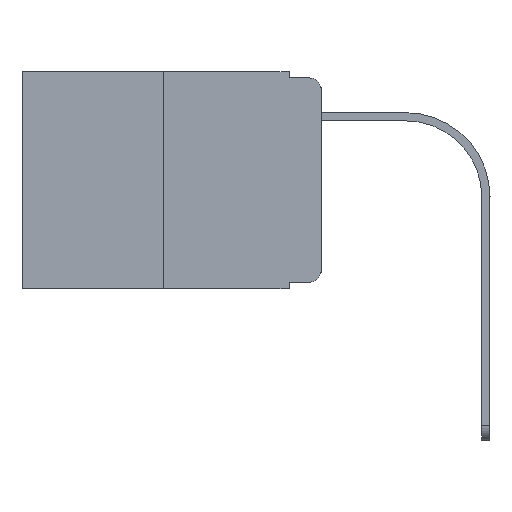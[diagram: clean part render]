
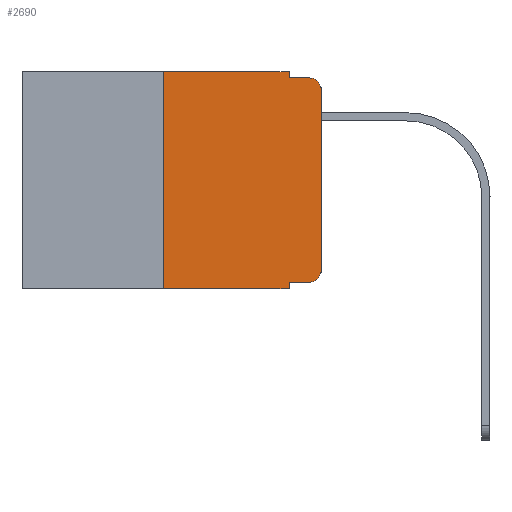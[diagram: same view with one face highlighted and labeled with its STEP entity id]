
A CAD part, left-side view. The second image highlights one B-rep face of the part: STEP entity #2690.
In plain terms, the highlighted planar face has unit normal (-1, 0, 0).
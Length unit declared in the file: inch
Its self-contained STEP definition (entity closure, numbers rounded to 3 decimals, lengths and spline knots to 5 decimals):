
#59 = CARTESIAN_POINT ( 'NONE',  ( 0., 0.051, 0. ) ) ;
#153 = DIRECTION ( 'NONE',  ( -1., 0., 0. ) ) ;
#318 = ORIENTED_EDGE ( 'NONE', *, *, #4493, .F. ) ;
#426 = CARTESIAN_POINT ( 'NONE',  ( 0., 0.473, 0. ) ) ;
#487 = DIRECTION ( 'NONE',  ( 1., 0., 0. ) ) ;
#497 = CIRCLE ( 'NONE', #7524, 0.02 ) ;
#690 = CARTESIAN_POINT ( 'NONE',  ( 0., 0.051, -0.01 ) ) ;
#861 = EDGE_CURVE ( 'NONE', #11144, #884, #11295, .T. ) ;
#884 = VERTEX_POINT ( 'NONE', #4668 ) ;
#1191 = EDGE_CURVE ( 'NONE', #9181, #11509, #8851, .T. ) ;
#1314 = ORIENTED_EDGE ( 'NONE', *, *, #3834, .F. ) ;
#1510 = VECTOR ( 'NONE', #5230, 39.37008 ) ;
#1540 = FACE_OUTER_BOUND ( 'NONE', #5552, .T. ) ;
#1610 = LINE ( 'NONE', #8327, #11600 ) ;
#1935 = ORIENTED_EDGE ( 'NONE', *, *, #7911, .T. ) ;
#2115 = DIRECTION ( 'NONE',  ( 0., 0., -1. ) ) ;
#2291 = LINE ( 'NONE', #8068, #1510 ) ;
#2505 = EDGE_CURVE ( 'NONE', #9447, #11509, #4619, .T. ) ;
#2646 = EDGE_CURVE ( 'NONE', #11144, #7673, #6015, .T. ) ;
#2681 = ORIENTED_EDGE ( 'NONE', *, *, #2850, .T. ) ;
#2690 = ADVANCED_FACE ( 'NONE', ( #1540 ), #9013, .F. ) ;
#2784 = CARTESIAN_POINT ( 'NONE',  ( 0., 0.25, 0. ) ) ;
#2837 = DIRECTION ( 'NONE',  ( 0., 0., -1. ) ) ;
#2850 = EDGE_CURVE ( 'NONE', #11468, #9181, #1610, .T. ) ;
#2859 = CARTESIAN_POINT ( 'NONE',  ( 0., 0., -0.313 ) ) ;
#2957 = CARTESIAN_POINT ( 'NONE',  ( 0., 0.051, 0. ) ) ;
#3092 = CARTESIAN_POINT ( 'NONE',  ( 0., 0.051, 0. ) ) ;
#3671 = ORIENTED_EDGE ( 'NONE', *, *, #1191, .T. ) ;
#3724 = CARTESIAN_POINT ( 'NONE',  ( 0., 0.25, -0.343 ) ) ;
#3834 = EDGE_CURVE ( 'NONE', #8949, #5104, #2291, .T. ) ;
#3927 = DIRECTION ( 'NONE',  ( 0., -1., 0. ) ) ;
#3936 = DIRECTION ( 'NONE',  ( 0., -1., 0. ) ) ;
#4010 = ORIENTED_EDGE ( 'NONE', *, *, #5837, .F. ) ;
#4493 = EDGE_CURVE ( 'NONE', #5104, #10825, #10637, .T. ) ;
#4619 = LINE ( 'NONE', #690, #6845 ) ;
#4668 = CARTESIAN_POINT ( 'NONE',  ( 0., 0.02, -0.333 ) ) ;
#4962 = VECTOR ( 'NONE', #2837, 39.37008 ) ;
#5104 = VERTEX_POINT ( 'NONE', #2784 ) ;
#5146 = DIRECTION ( 'NONE',  ( 0., 0., -1. ) ) ;
#5230 = DIRECTION ( 'NONE',  ( 0., 0., 1. ) ) ;
#5240 = DIRECTION ( 'NONE',  ( 0., 0., -1. ) ) ;
#5477 = ORIENTED_EDGE ( 'NONE', *, *, #6198, .T. ) ;
#5552 = EDGE_LOOP ( 'NONE', ( #2681, #3671, #10069, #4010, #318, #1314, #5477, #10979, #10586, #1935 ) ) ;
#5634 = DIRECTION ( 'NONE',  ( 0., -1., 0. ) ) ;
#5811 = CARTESIAN_POINT ( 'NONE',  ( 0., 0.02, -0.01 ) ) ;
#5837 = EDGE_CURVE ( 'NONE', #10825, #9447, #11525, .T. ) ;
#5990 = VECTOR ( 'NONE', #3927, 39.37008 ) ;
#6015 = LINE ( 'NONE', #59, #7045 ) ;
#6198 = EDGE_CURVE ( 'NONE', #8949, #7673, #10458, .T. ) ;
#6517 = DIRECTION ( 'NONE',  ( 0., -1., 0. ) ) ;
#6740 = VECTOR ( 'NONE', #3936, 39.37008 ) ;
#6845 = VECTOR ( 'NONE', #5634, 39.37008 ) ;
#7017 = CARTESIAN_POINT ( 'NONE',  ( 0., 0.051, -0.343 ) ) ;
#7045 = VECTOR ( 'NONE', #2115, 39.37008 ) ;
#7294 = VECTOR ( 'NONE', #6517, 39.37008 ) ;
#7524 = AXIS2_PLACEMENT_3D ( 'NONE', #10475, #153, #5146 ) ;
#7673 = VERTEX_POINT ( 'NONE', #7017 ) ;
#7911 = EDGE_CURVE ( 'NONE', #884, #11468, #497, .T. ) ;
#8068 = CARTESIAN_POINT ( 'NONE',  ( 0., 0.25, 0. ) ) ;
#8224 = AXIS2_PLACEMENT_3D ( 'NONE', #426, #487, #5240 ) ;
#8327 = CARTESIAN_POINT ( 'NONE',  ( 0., 0., 0. ) ) ;
#8390 = DIRECTION ( 'NONE',  ( 0., 0., 1. ) ) ;
#8506 = CARTESIAN_POINT ( 'NONE',  ( 0., 0.02, -0.03 ) ) ;
#8851 = CIRCLE ( 'NONE', #11613, 0.02 ) ;
#8949 = VERTEX_POINT ( 'NONE', #3724 ) ;
#9013 = PLANE ( 'NONE',  #8224 ) ;
#9181 = VERTEX_POINT ( 'NONE', #10788 ) ;
#9238 = CARTESIAN_POINT ( 'NONE',  ( 0., 0.051, -0.01 ) ) ;
#9447 = VERTEX_POINT ( 'NONE', #9238 ) ;
#9548 = DIRECTION ( 'NONE',  ( -1., 0., 0. ) ) ;
#9713 = CARTESIAN_POINT ( 'NONE',  ( 0., 0.051, -0.333 ) ) ;
#10069 = ORIENTED_EDGE ( 'NONE', *, *, #2505, .F. ) ;
#10458 = LINE ( 'NONE', #12315, #5990 ) ;
#10475 = CARTESIAN_POINT ( 'NONE',  ( 0., 0.02, -0.313 ) ) ;
#10586 = ORIENTED_EDGE ( 'NONE', *, *, #861, .T. ) ;
#10637 = LINE ( 'NONE', #11640, #6740 ) ;
#10788 = CARTESIAN_POINT ( 'NONE',  ( 0., 0., -0.03 ) ) ;
#10825 = VERTEX_POINT ( 'NONE', #3092 ) ;
#10979 = ORIENTED_EDGE ( 'NONE', *, *, #2646, .F. ) ;
#11144 = VERTEX_POINT ( 'NONE', #9713 ) ;
#11295 = LINE ( 'NONE', #11427, #7294 ) ;
#11340 = DIRECTION ( 'NONE',  ( 0., 0., -1. ) ) ;
#11427 = CARTESIAN_POINT ( 'NONE',  ( 0., 0.051, -0.333 ) ) ;
#11468 = VERTEX_POINT ( 'NONE', #2859 ) ;
#11509 = VERTEX_POINT ( 'NONE', #5811 ) ;
#11525 = LINE ( 'NONE', #2957, #4962 ) ;
#11600 = VECTOR ( 'NONE', #8390, 39.37008 ) ;
#11613 = AXIS2_PLACEMENT_3D ( 'NONE', #8506, #9548, #11340 ) ;
#11640 = CARTESIAN_POINT ( 'NONE',  ( 0., 0.473, 0. ) ) ;
#12315 = CARTESIAN_POINT ( 'NONE',  ( 0., 0.473, -0.343 ) ) ;
